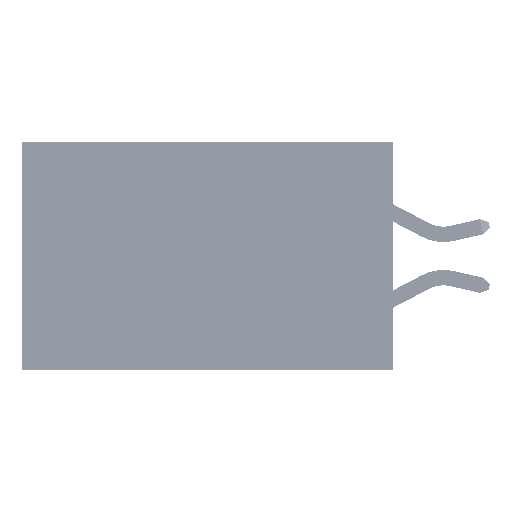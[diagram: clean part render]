
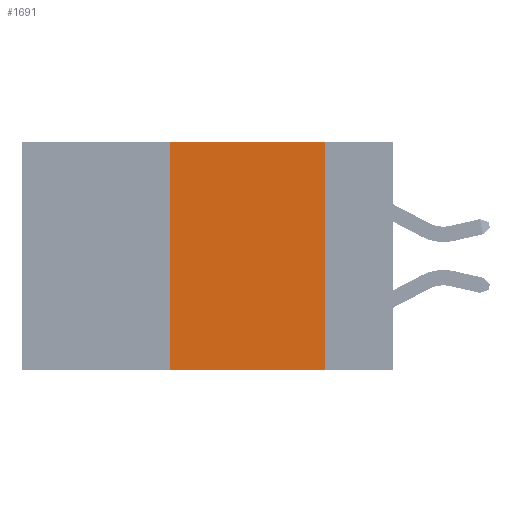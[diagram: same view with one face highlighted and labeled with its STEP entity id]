
A CAD part, left-side view. The second image highlights one B-rep face of the part: STEP entity #1691.
In plain terms, the highlighted planar face has unit normal (-1, 0, 0).
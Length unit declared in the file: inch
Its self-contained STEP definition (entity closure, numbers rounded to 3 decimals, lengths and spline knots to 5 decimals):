
#1260 = DIRECTION ( 'NONE',  ( 0., -1., 0. ) ) ;
#1691 = ADVANCED_FACE ( 'NONE', ( #14309 ), #37008, .F. ) ;
#2212 = LINE ( 'NONE', #17441, #22143 ) ;
#3790 = EDGE_CURVE ( 'NONE', #38622, #16504, #30450, .T. ) ;
#5363 = VECTOR ( 'NONE', #11961, 39.37008 ) ;
#6511 = ORIENTED_EDGE ( 'NONE', *, *, #30704, .T. ) ;
#10039 = VECTOR ( 'NONE', #1260, 39.37008 ) ;
#10063 = DIRECTION ( 'NONE',  ( 1., 0., 0. ) ) ;
#11961 = DIRECTION ( 'NONE',  ( 0., 0., -1. ) ) ;
#13609 = VECTOR ( 'NONE', #16234, 39.37008 ) ;
#14309 = FACE_OUTER_BOUND ( 'NONE', #43238, .T. ) ;
#16234 = DIRECTION ( 'NONE',  ( 0., 0., 1. ) ) ;
#16504 = VERTEX_POINT ( 'NONE', #42315 ) ;
#17441 = CARTESIAN_POINT ( 'NONE',  ( 0., 0.6, -0.37 ) ) ;
#18056 = ORIENTED_EDGE ( 'NONE', *, *, #42681, .F. ) ;
#18721 = VERTEX_POINT ( 'NONE', #29627 ) ;
#19195 = ORIENTED_EDGE ( 'NONE', *, *, #28817, .F. ) ;
#19202 = CARTESIAN_POINT ( 'NONE',  ( 0., 0.11, 0. ) ) ;
#20742 = LINE ( 'NONE', #43470, #10039 ) ;
#21920 = DIRECTION ( 'NONE',  ( 0., -1., 0. ) ) ;
#22143 = VECTOR ( 'NONE', #21920, 39.37008 ) ;
#24457 = CARTESIAN_POINT ( 'NONE',  ( 0., 0.36, -0.37 ) ) ;
#24794 = DIRECTION ( 'NONE',  ( 0., 0., -1. ) ) ;
#28817 = EDGE_CURVE ( 'NONE', #16504, #18721, #20742, .T. ) ;
#29498 = VERTEX_POINT ( 'NONE', #36887 ) ;
#29627 = CARTESIAN_POINT ( 'NONE',  ( 0., 0.11, 0. ) ) ;
#30450 = LINE ( 'NONE', #45718, #13609 ) ;
#30704 = EDGE_CURVE ( 'NONE', #38622, #29498, #2212, .T. ) ;
#34171 = LINE ( 'NONE', #19202, #5363 ) ;
#36770 = CARTESIAN_POINT ( 'NONE',  ( 0., 0.6, 0. ) ) ;
#36887 = CARTESIAN_POINT ( 'NONE',  ( 0., 0.11, -0.37 ) ) ;
#37008 = PLANE ( 'NONE',  #45095 ) ;
#38622 = VERTEX_POINT ( 'NONE', #24457 ) ;
#42315 = CARTESIAN_POINT ( 'NONE',  ( 0., 0.36, 0. ) ) ;
#42681 = EDGE_CURVE ( 'NONE', #18721, #29498, #34171, .T. ) ;
#43238 = EDGE_LOOP ( 'NONE', ( #18056, #19195, #45674, #6511 ) ) ;
#43470 = CARTESIAN_POINT ( 'NONE',  ( 0., 0.6, 0. ) ) ;
#45095 = AXIS2_PLACEMENT_3D ( 'NONE', #36770, #10063, #24794 ) ;
#45674 = ORIENTED_EDGE ( 'NONE', *, *, #3790, .F. ) ;
#45718 = CARTESIAN_POINT ( 'NONE',  ( 0., 0.36, 0. ) ) ;
